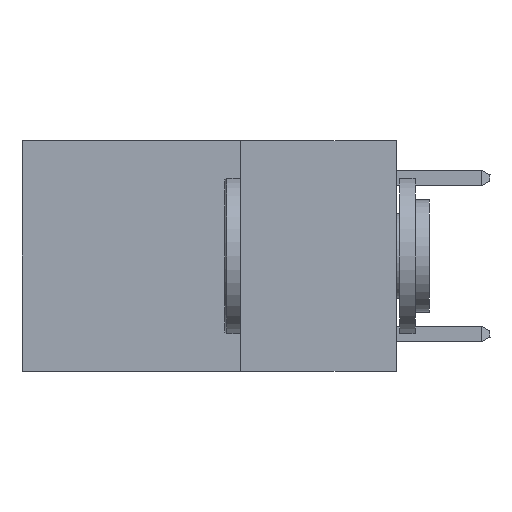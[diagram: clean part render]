
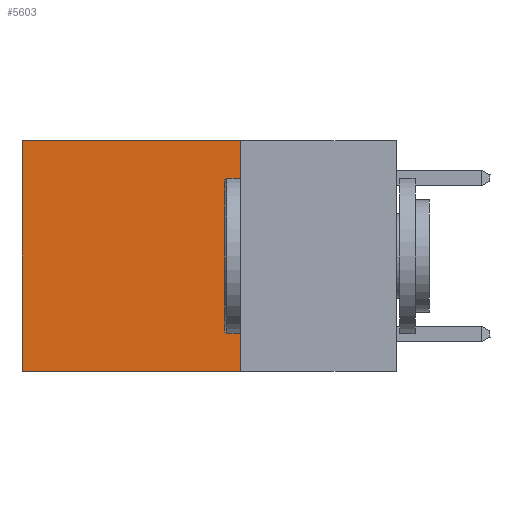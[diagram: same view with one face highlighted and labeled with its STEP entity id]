
A CAD part, left-side view. The second image highlights one B-rep face of the part: STEP entity #5603.
In plain terms, the highlighted planar face has unit normal (-1, 0, 0).
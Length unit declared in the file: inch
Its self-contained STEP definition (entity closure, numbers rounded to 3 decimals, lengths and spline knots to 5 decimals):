
#108 = ORIENTED_EDGE ( 'NONE', *, *, #18236, .F. ) ;
#437 = CARTESIAN_POINT ( 'NONE',  ( 0.2625, 0.6, -0.37 ) ) ;
#528 = LINE ( 'NONE', #19778, #19636 ) ;
#974 = EDGE_LOOP ( 'NONE', ( #10750, #21745, #108, #18892 ) ) ;
#1024 = CARTESIAN_POINT ( 'NONE',  ( 0.2625, 0.25, 0. ) ) ;
#1602 = CARTESIAN_POINT ( 'NONE',  ( 0.2625, 0.6, 0. ) ) ;
#5603 = ADVANCED_FACE ( 'NONE', ( #11494 ), #19173, .F. ) ;
#5899 = VERTEX_POINT ( 'NONE', #13317 ) ;
#6402 = DIRECTION ( 'NONE',  ( 0., 0., -1. ) ) ;
#7859 = DIRECTION ( 'NONE',  ( 1., 0., 0. ) ) ;
#8550 = VECTOR ( 'NONE', #6402, 39.37008 ) ;
#8803 = VERTEX_POINT ( 'NONE', #1602 ) ;
#8863 = LINE ( 'NONE', #23865, #24664 ) ;
#9356 = LINE ( 'NONE', #15140, #19944 ) ;
#10212 = DIRECTION ( 'NONE',  ( 0., 1., 0. ) ) ;
#10750 = ORIENTED_EDGE ( 'NONE', *, *, #18056, .T. ) ;
#10756 = VERTEX_POINT ( 'NONE', #437 ) ;
#11494 = FACE_OUTER_BOUND ( 'NONE', #974, .T. ) ;
#13317 = CARTESIAN_POINT ( 'NONE',  ( 0.2625, 0.25, -0.37 ) ) ;
#13887 = CARTESIAN_POINT ( 'NONE',  ( 0.2625, 0.25, 0. ) ) ;
#14437 = EDGE_CURVE ( 'NONE', #5899, #10756, #9356, .T. ) ;
#14645 = VERTEX_POINT ( 'NONE', #1024 ) ;
#15140 = CARTESIAN_POINT ( 'NONE',  ( 0.2625, 0.25, -0.37 ) ) ;
#15403 = DIRECTION ( 'NONE',  ( 0., 0., -1. ) ) ;
#15821 = EDGE_CURVE ( 'NONE', #14645, #8803, #528, .T. ) ;
#16224 = LINE ( 'NONE', #23803, #8550 ) ;
#16411 = DIRECTION ( 'NONE',  ( 0., 0., -1. ) ) ;
#18056 = EDGE_CURVE ( 'NONE', #8803, #10756, #8863, .T. ) ;
#18236 = EDGE_CURVE ( 'NONE', #14645, #5899, #16224, .T. ) ;
#18892 = ORIENTED_EDGE ( 'NONE', *, *, #15821, .T. ) ;
#19173 = PLANE ( 'NONE',  #24304 ) ;
#19636 = VECTOR ( 'NONE', #10212, 39.37008 ) ;
#19778 = CARTESIAN_POINT ( 'NONE',  ( 0.2625, 0.25, 0. ) ) ;
#19944 = VECTOR ( 'NONE', #22853, 39.37008 ) ;
#21745 = ORIENTED_EDGE ( 'NONE', *, *, #14437, .F. ) ;
#22853 = DIRECTION ( 'NONE',  ( 0., 1., 0. ) ) ;
#23803 = CARTESIAN_POINT ( 'NONE',  ( 0.2625, 0.25, 0. ) ) ;
#23865 = CARTESIAN_POINT ( 'NONE',  ( 0.2625, 0.6, 0. ) ) ;
#24304 = AXIS2_PLACEMENT_3D ( 'NONE', #13887, #7859, #15403 ) ;
#24664 = VECTOR ( 'NONE', #16411, 39.37008 ) ;
